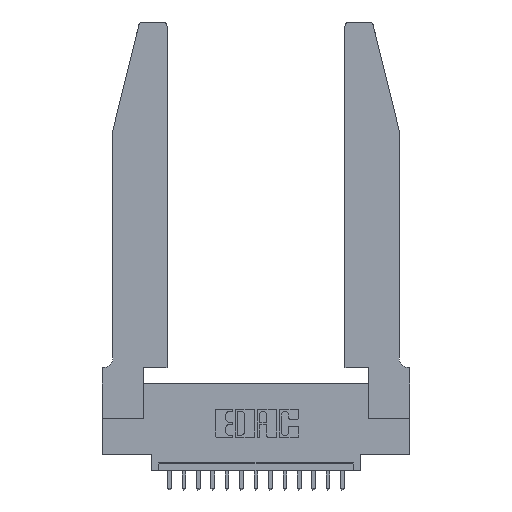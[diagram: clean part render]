
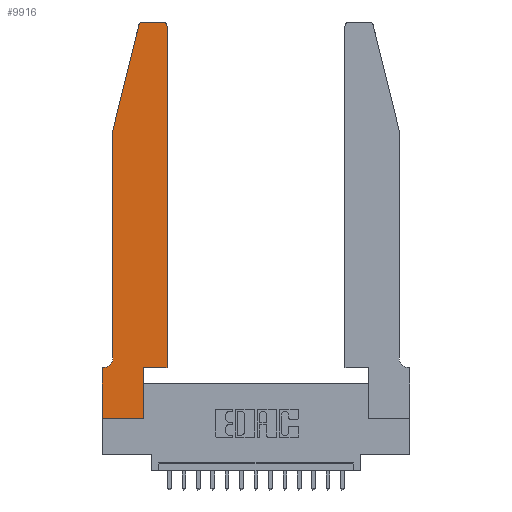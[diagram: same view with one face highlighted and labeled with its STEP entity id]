
A CAD part, top view. The second image highlights one B-rep face of the part: STEP entity #9916.
In plain terms, the highlighted planar face has unit normal (0, 0, 1).
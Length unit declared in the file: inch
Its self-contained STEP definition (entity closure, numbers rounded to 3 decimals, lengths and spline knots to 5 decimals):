
#89 = CARTESIAN_POINT ( 'NONE',  ( 0., 0., 0.37 ) ) ;
#324 = CARTESIAN_POINT ( 'NONE',  ( 0.2865, 0.35, 0.37 ) ) ;
#485 = CARTESIAN_POINT ( 'NONE',  ( 0.4205, 2.75, 0.37 ) ) ;
#916 = LINE ( 'NONE', #9822, #11952 ) ;
#932 = DIRECTION ( 'NONE',  ( 0., 0., 1. ) ) ;
#933 = ORIENTED_EDGE ( 'NONE', *, *, #2666, .T. ) ;
#995 = FACE_OUTER_BOUND ( 'NONE', #13665, .T. ) ;
#1192 = PLANE ( 'NONE',  #1507 ) ;
#1507 = AXIS2_PLACEMENT_3D ( 'NONE', #2656, #932, #18387 ) ;
#1564 = LINE ( 'NONE', #3116, #8087 ) ;
#1747 = CARTESIAN_POINT ( 'NONE',  ( 0.284, 2.75, 0.37 ) ) ;
#1829 = LINE ( 'NONE', #6958, #18452 ) ;
#2062 = ORIENTED_EDGE ( 'NONE', *, *, #16143, .T. ) ;
#2243 = ORIENTED_EDGE ( 'NONE', *, *, #11802, .T. ) ;
#2505 = DIRECTION ( 'NONE',  ( -1., 0., 0. ) ) ;
#2604 = AXIS2_PLACEMENT_3D ( 'NONE', #5333, #15507, #18337 ) ;
#2656 = CARTESIAN_POINT ( 'NONE',  ( 0., 0.35, 0.37 ) ) ;
#2666 = EDGE_CURVE ( 'NONE', #3883, #6804, #13610, .T. ) ;
#2926 = VERTEX_POINT ( 'NONE', #5634 ) ;
#2933 = EDGE_CURVE ( 'NONE', #8439, #6741, #12716, .T. ) ;
#3047 = EDGE_CURVE ( 'NONE', #17734, #3883, #18085, .T. ) ;
#3116 = CARTESIAN_POINT ( 'NONE',  ( 0.2865, 0.35, 0.37 ) ) ;
#3281 = VECTOR ( 'NONE', #7015, 39.37008 ) ;
#3666 = VERTEX_POINT ( 'NONE', #7715 ) ;
#3883 = VERTEX_POINT ( 'NONE', #18274 ) ;
#4728 = DIRECTION ( 'NONE',  ( 0., 1., 0. ) ) ;
#5126 = LINE ( 'NONE', #6225, #16141 ) ;
#5333 = CARTESIAN_POINT ( 'NONE',  ( 0.4205, 2.72, 0.37 ) ) ;
#5382 = CARTESIAN_POINT ( 'NONE',  ( 0.2605, 2.75, 0.37 ) ) ;
#5399 = ORIENTED_EDGE ( 'NONE', *, *, #18560, .T. ) ;
#5461 = CARTESIAN_POINT ( 'NONE',  ( 0.0755, 2., 0.37 ) ) ;
#5462 = CARTESIAN_POINT ( 'NONE',  ( 0.2865, 0., 0.37 ) ) ;
#5634 = CARTESIAN_POINT ( 'NONE',  ( 0., 0., 0.37 ) ) ;
#5976 = DIRECTION ( 'NONE',  ( 0., -1., 0. ) ) ;
#6043 = CIRCLE ( 'NONE', #13631, 0.07 ) ;
#6072 = CARTESIAN_POINT ( 'NONE',  ( 0.0755, 2., 0.37 ) ) ;
#6225 = CARTESIAN_POINT ( 'NONE',  ( 0., 0., 0.37 ) ) ;
#6741 = VERTEX_POINT ( 'NONE', #13773 ) ;
#6804 = VERTEX_POINT ( 'NONE', #5461 ) ;
#6849 = LINE ( 'NONE', #89, #18543 ) ;
#6853 = ORIENTED_EDGE ( 'NONE', *, *, #3047, .T. ) ;
#6958 = CARTESIAN_POINT ( 'NONE',  ( 0.0755, 0.35, 0.37 ) ) ;
#6967 = EDGE_CURVE ( 'NONE', #11628, #7593, #1564, .T. ) ;
#7015 = DIRECTION ( 'NONE',  ( -0.239, -0.971, 0. ) ) ;
#7457 = ORIENTED_EDGE ( 'NONE', *, *, #12140, .T. ) ;
#7593 = VERTEX_POINT ( 'NONE', #324 ) ;
#7626 = CARTESIAN_POINT ( 'NONE',  ( 0.4505, 0.35, 0.37 ) ) ;
#7715 = CARTESIAN_POINT ( 'NONE',  ( 0.0755, 0.42, 0.37 ) ) ;
#7898 = DIRECTION ( 'NONE',  ( -1., 0., 0. ) ) ;
#8087 = VECTOR ( 'NONE', #13182, 39.37008 ) ;
#8114 = VECTOR ( 'NONE', #8680, 39.37008 ) ;
#8231 = DIRECTION ( 'NONE',  ( 1., 0., 0. ) ) ;
#8257 = DIRECTION ( 'NONE',  ( -1., 0., 0. ) ) ;
#8439 = VERTEX_POINT ( 'NONE', #7626 ) ;
#8504 = LINE ( 'NONE', #5382, #12966 ) ;
#8598 = DIRECTION ( 'NONE',  ( 1., 0., 0. ) ) ;
#8680 = DIRECTION ( 'NONE',  ( 0., -1., 0. ) ) ;
#8712 = EDGE_CURVE ( 'NONE', #6741, #11382, #12968, .T. ) ;
#8788 = VERTEX_POINT ( 'NONE', #17028 ) ;
#9235 = VERTEX_POINT ( 'NONE', #9261 ) ;
#9261 = CARTESIAN_POINT ( 'NONE',  ( 0., 0.35, 0.37 ) ) ;
#9313 = DIRECTION ( 'NONE',  ( 0., 0., -1. ) ) ;
#9440 = ORIENTED_EDGE ( 'NONE', *, *, #11837, .T. ) ;
#9822 = CARTESIAN_POINT ( 'NONE',  ( 0.4505, 0.35, 0.37 ) ) ;
#9916 = ADVANCED_FACE ( 'NONE', ( #995 ), #1192, .T. ) ;
#10808 = CARTESIAN_POINT ( 'NONE',  ( 0.0055, 0.42, 0.37 ) ) ;
#11382 = VERTEX_POINT ( 'NONE', #485 ) ;
#11628 = VERTEX_POINT ( 'NONE', #5462 ) ;
#11802 = EDGE_CURVE ( 'NONE', #8788, #9235, #1829, .T. ) ;
#11837 = EDGE_CURVE ( 'NONE', #7593, #8439, #916, .T. ) ;
#11952 = VECTOR ( 'NONE', #8231, 39.37008 ) ;
#12140 = EDGE_CURVE ( 'NONE', #6804, #3666, #17542, .T. ) ;
#12477 = VECTOR ( 'NONE', #4728, 39.37008 ) ;
#12561 = CARTESIAN_POINT ( 'NONE',  ( 0.284, 2.72, 0.37 ) ) ;
#12716 = LINE ( 'NONE', #13061, #12477 ) ;
#12966 = VECTOR ( 'NONE', #8257, 39.37008 ) ;
#12968 = CIRCLE ( 'NONE', #2604, 0.03 ) ;
#13061 = CARTESIAN_POINT ( 'NONE',  ( 0.4505, 0.35, 0.37 ) ) ;
#13182 = DIRECTION ( 'NONE',  ( 0., 1., 0. ) ) ;
#13610 = LINE ( 'NONE', #16475, #3281 ) ;
#13631 = AXIS2_PLACEMENT_3D ( 'NONE', #10808, #9313, #7898 ) ;
#13665 = EDGE_LOOP ( 'NONE', ( #13811, #6853, #933, #7457, #2062, #2243, #14893, #5399, #17559, #9440, #17067, #18500 ) ) ;
#13773 = CARTESIAN_POINT ( 'NONE',  ( 0.4505, 2.72, 0.37 ) ) ;
#13811 = ORIENTED_EDGE ( 'NONE', *, *, #17463, .T. ) ;
#14017 = DIRECTION ( 'NONE',  ( 0., 0., 1. ) ) ;
#14158 = EDGE_CURVE ( 'NONE', #9235, #2926, #5126, .T. ) ;
#14893 = ORIENTED_EDGE ( 'NONE', *, *, #14158, .T. ) ;
#15507 = DIRECTION ( 'NONE',  ( 0., 0., 1. ) ) ;
#15569 = DIRECTION ( 'NONE',  ( 1., 0., 0. ) ) ;
#15673 = AXIS2_PLACEMENT_3D ( 'NONE', #12561, #14017, #15569 ) ;
#16141 = VECTOR ( 'NONE', #5976, 39.37008 ) ;
#16143 = EDGE_CURVE ( 'NONE', #3666, #8788, #6043, .T. ) ;
#16475 = CARTESIAN_POINT ( 'NONE',  ( 0.0755, 2., 0.37 ) ) ;
#17028 = CARTESIAN_POINT ( 'NONE',  ( 0.0055, 0.35, 0.37 ) ) ;
#17067 = ORIENTED_EDGE ( 'NONE', *, *, #2933, .T. ) ;
#17463 = EDGE_CURVE ( 'NONE', #11382, #17734, #8504, .T. ) ;
#17542 = LINE ( 'NONE', #6072, #8114 ) ;
#17559 = ORIENTED_EDGE ( 'NONE', *, *, #6967, .T. ) ;
#17734 = VERTEX_POINT ( 'NONE', #1747 ) ;
#18085 = CIRCLE ( 'NONE', #15673, 0.03 ) ;
#18274 = CARTESIAN_POINT ( 'NONE',  ( 0.25487, 2.72718, 0.37 ) ) ;
#18337 = DIRECTION ( 'NONE',  ( 1., 0., 0. ) ) ;
#18387 = DIRECTION ( 'NONE',  ( 1., 0., 0. ) ) ;
#18452 = VECTOR ( 'NONE', #2505, 39.37008 ) ;
#18500 = ORIENTED_EDGE ( 'NONE', *, *, #8712, .T. ) ;
#18543 = VECTOR ( 'NONE', #8598, 39.37008 ) ;
#18560 = EDGE_CURVE ( 'NONE', #2926, #11628, #6849, .T. ) ;
